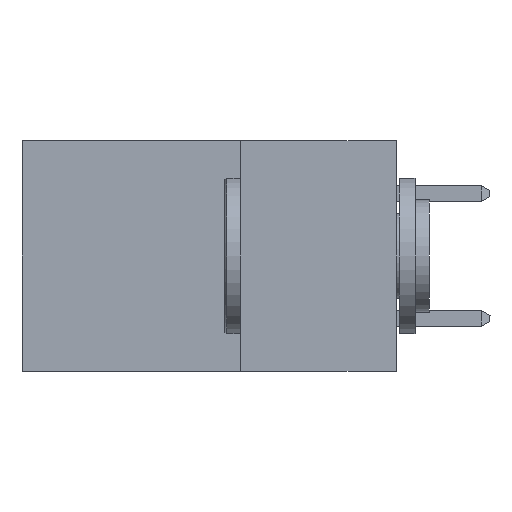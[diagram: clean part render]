
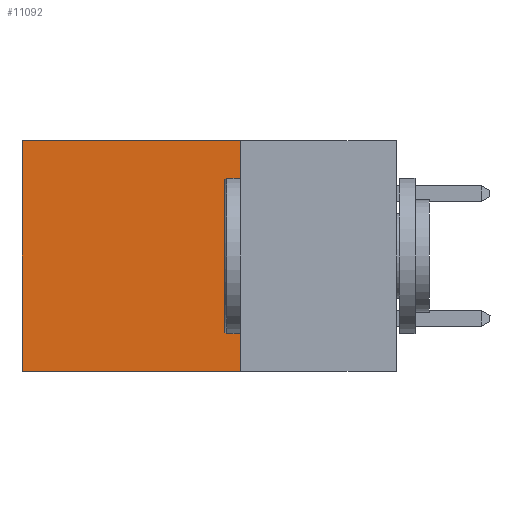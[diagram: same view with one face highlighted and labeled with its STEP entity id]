
A CAD part, left-side view. The second image highlights one B-rep face of the part: STEP entity #11092.
In plain terms, the highlighted planar face has unit normal (-1, 0, 0).
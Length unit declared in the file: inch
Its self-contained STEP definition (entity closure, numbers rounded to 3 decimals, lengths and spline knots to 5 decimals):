
#343 = VERTEX_POINT ( 'NONE', #3777 ) ;
#462 = VERTEX_POINT ( 'NONE', #5219 ) ;
#780 = DIRECTION ( 'NONE',  ( 0., 1., 0. ) ) ;
#1278 = VECTOR ( 'NONE', #12536, 39.37008 ) ;
#1372 = DIRECTION ( 'NONE',  ( 0., 0., -1. ) ) ;
#1893 = CARTESIAN_POINT ( 'NONE',  ( 0.298, 0.6, -0.37 ) ) ;
#2183 = ORIENTED_EDGE ( 'NONE', *, *, #10256, .F. ) ;
#2502 = VECTOR ( 'NONE', #1372, 39.37008 ) ;
#2739 = VERTEX_POINT ( 'NONE', #1893 ) ;
#3186 = CARTESIAN_POINT ( 'NONE',  ( 0.298, 0.25, -0.37 ) ) ;
#3231 = ORIENTED_EDGE ( 'NONE', *, *, #10437, .F. ) ;
#3466 = LINE ( 'NONE', #3186, #7400 ) ;
#3686 = VECTOR ( 'NONE', #780, 39.37008 ) ;
#3777 = CARTESIAN_POINT ( 'NONE',  ( 0.298, 0.25, 0. ) ) ;
#4285 = DIRECTION ( 'NONE',  ( 0., 0., -1. ) ) ;
#4329 = CARTESIAN_POINT ( 'NONE',  ( 0.298, 0.25, 0. ) ) ;
#4668 = FACE_OUTER_BOUND ( 'NONE', #6628, .T. ) ;
#4961 = ORIENTED_EDGE ( 'NONE', *, *, #12064, .T. ) ;
#5219 = CARTESIAN_POINT ( 'NONE',  ( 0.298, 0.25, -0.37 ) ) ;
#5757 = LINE ( 'NONE', #10218, #1278 ) ;
#6628 = EDGE_LOOP ( 'NONE', ( #4961, #2183, #3231, #7875 ) ) ;
#7400 = VECTOR ( 'NONE', #11745, 39.37008 ) ;
#7875 = ORIENTED_EDGE ( 'NONE', *, *, #12708, .T. ) ;
#9124 = VERTEX_POINT ( 'NONE', #10804 ) ;
#10055 = LINE ( 'NONE', #13012, #3686 ) ;
#10158 = LINE ( 'NONE', #11650, #2502 ) ;
#10218 = CARTESIAN_POINT ( 'NONE',  ( 0.298, 0.6, 0. ) ) ;
#10256 = EDGE_CURVE ( 'NONE', #462, #2739, #3466, .T. ) ;
#10437 = EDGE_CURVE ( 'NONE', #343, #462, #10158, .T. ) ;
#10804 = CARTESIAN_POINT ( 'NONE',  ( 0.298, 0.6, 0. ) ) ;
#11092 = ADVANCED_FACE ( 'NONE', ( #4668 ), #11524, .F. ) ;
#11524 = PLANE ( 'NONE',  #12857 ) ;
#11650 = CARTESIAN_POINT ( 'NONE',  ( 0.298, 0.25, 0. ) ) ;
#11745 = DIRECTION ( 'NONE',  ( 0., 1., 0. ) ) ;
#12064 = EDGE_CURVE ( 'NONE', #9124, #2739, #5757, .T. ) ;
#12423 = DIRECTION ( 'NONE',  ( 1., 0., 0. ) ) ;
#12536 = DIRECTION ( 'NONE',  ( 0., 0., -1. ) ) ;
#12708 = EDGE_CURVE ( 'NONE', #343, #9124, #10055, .T. ) ;
#12857 = AXIS2_PLACEMENT_3D ( 'NONE', #4329, #12423, #4285 ) ;
#13012 = CARTESIAN_POINT ( 'NONE',  ( 0.298, 0.25, 0. ) ) ;
